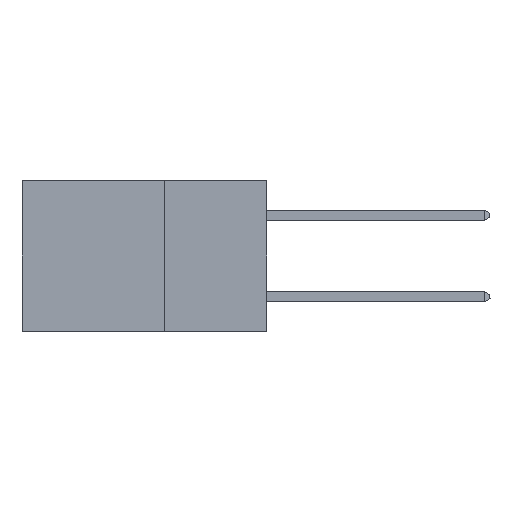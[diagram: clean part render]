
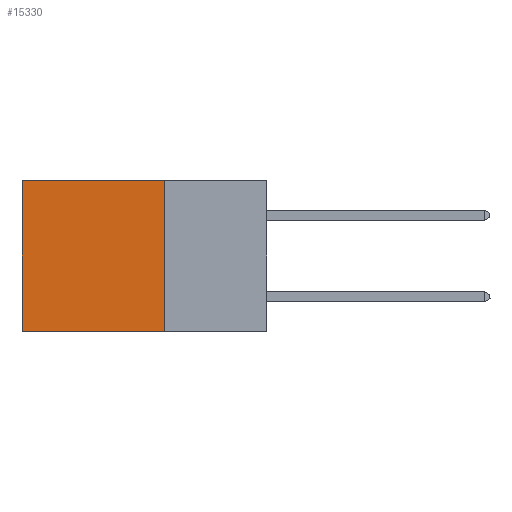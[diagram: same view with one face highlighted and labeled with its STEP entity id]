
A CAD part, left-side view. The second image highlights one B-rep face of the part: STEP entity #15330.
In plain terms, the highlighted planar face has unit normal (-1, 0, 0).
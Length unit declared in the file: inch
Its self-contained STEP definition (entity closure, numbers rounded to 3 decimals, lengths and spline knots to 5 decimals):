
#358 = DIRECTION ( 'NONE',  ( 0., 1., 0. ) ) ;
#420 = VERTEX_POINT ( 'NONE', #10945 ) ;
#623 = VECTOR ( 'NONE', #12980, 39.37008 ) ;
#812 = LINE ( 'NONE', #20050, #6392 ) ;
#1488 = LINE ( 'NONE', #12066, #623 ) ;
#3970 = CARTESIAN_POINT ( 'NONE',  ( 0.2875, 0.25, 0. ) ) ;
#5083 = EDGE_CURVE ( 'NONE', #420, #15675, #1488, .T. ) ;
#5131 = CARTESIAN_POINT ( 'NONE',  ( 0.2875, 0.25, -0.37 ) ) ;
#6098 = VERTEX_POINT ( 'NONE', #10811 ) ;
#6392 = VECTOR ( 'NONE', #358, 39.37008 ) ;
#8924 = ORIENTED_EDGE ( 'NONE', *, *, #5083, .F. ) ;
#9078 = VECTOR ( 'NONE', #18201, 39.37008 ) ;
#9879 = CARTESIAN_POINT ( 'NONE',  ( 0.2875, 0.6, -0.37 ) ) ;
#10811 = CARTESIAN_POINT ( 'NONE',  ( 0.2875, 0.6, 0. ) ) ;
#10945 = CARTESIAN_POINT ( 'NONE',  ( 0.2875, 0.25, 0. ) ) ;
#11450 = PLANE ( 'NONE',  #16782 ) ;
#11729 = VECTOR ( 'NONE', #13660, 39.37008 ) ;
#12066 = CARTESIAN_POINT ( 'NONE',  ( 0.2875, 0.25, 0. ) ) ;
#12980 = DIRECTION ( 'NONE',  ( 0., 0., -1. ) ) ;
#13660 = DIRECTION ( 'NONE',  ( 0., 0., -1. ) ) ;
#13743 = CARTESIAN_POINT ( 'NONE',  ( 0.2875, 0.6, 0. ) ) ;
#14076 = EDGE_CURVE ( 'NONE', #6098, #21067, #16527, .T. ) ;
#14439 = LINE ( 'NONE', #23119, #9078 ) ;
#14601 = ORIENTED_EDGE ( 'NONE', *, *, #20247, .F. ) ;
#15330 = ADVANCED_FACE ( 'NONE', ( #18593 ), #11450, .F. ) ;
#15675 = VERTEX_POINT ( 'NONE', #5131 ) ;
#16204 = ORIENTED_EDGE ( 'NONE', *, *, #17248, .T. ) ;
#16527 = LINE ( 'NONE', #13743, #11729 ) ;
#16663 = DIRECTION ( 'NONE',  ( 1., 0., 0. ) ) ;
#16782 = AXIS2_PLACEMENT_3D ( 'NONE', #3970, #16663, #20185 ) ;
#17248 = EDGE_CURVE ( 'NONE', #420, #6098, #812, .T. ) ;
#17627 = ORIENTED_EDGE ( 'NONE', *, *, #14076, .T. ) ;
#18201 = DIRECTION ( 'NONE',  ( 0., 1., 0. ) ) ;
#18434 = EDGE_LOOP ( 'NONE', ( #17627, #14601, #8924, #16204 ) ) ;
#18593 = FACE_OUTER_BOUND ( 'NONE', #18434, .T. ) ;
#20050 = CARTESIAN_POINT ( 'NONE',  ( 0.2875, 0.25, 0. ) ) ;
#20185 = DIRECTION ( 'NONE',  ( 0., 0., -1. ) ) ;
#20247 = EDGE_CURVE ( 'NONE', #15675, #21067, #14439, .T. ) ;
#21067 = VERTEX_POINT ( 'NONE', #9879 ) ;
#23119 = CARTESIAN_POINT ( 'NONE',  ( 0.2875, 0.25, -0.37 ) ) ;
